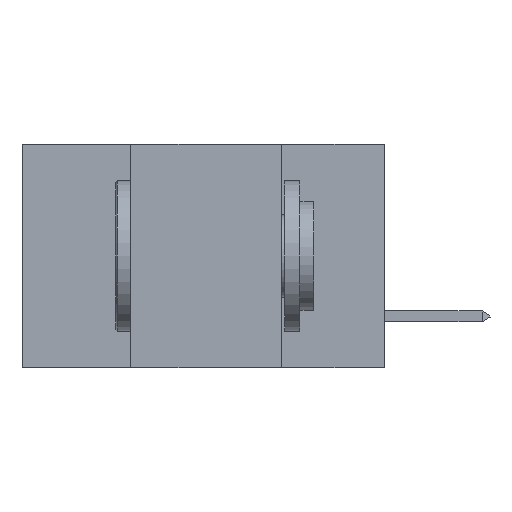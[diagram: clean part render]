
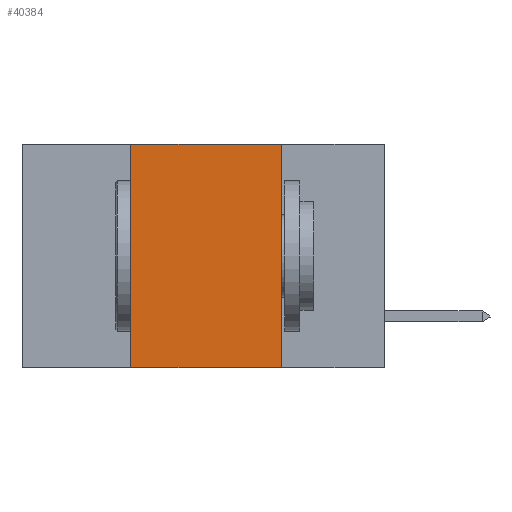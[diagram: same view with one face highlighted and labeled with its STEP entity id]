
A CAD part, left-side view. The second image highlights one B-rep face of the part: STEP entity #40384.
In plain terms, the highlighted planar face has unit normal (-1, 0, 0).
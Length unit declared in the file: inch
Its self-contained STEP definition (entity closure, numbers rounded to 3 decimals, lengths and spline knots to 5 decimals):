
#742 = ORIENTED_EDGE ( 'NONE', *, *, #41361, .F. ) ;
#785 = EDGE_LOOP ( 'NONE', ( #19359, #10120, #742, #43513 ) ) ;
#1730 = CARTESIAN_POINT ( 'NONE',  ( 0., 0.42, -0.37 ) ) ;
#3085 = LINE ( 'NONE', #10247, #39318 ) ;
#8878 = CARTESIAN_POINT ( 'NONE',  ( 0., 0.17, 0. ) ) ;
#9222 = DIRECTION ( 'NONE',  ( 0., -1., 0. ) ) ;
#9791 = VECTOR ( 'NONE', #37718, 39.37008 ) ;
#10120 = ORIENTED_EDGE ( 'NONE', *, *, #30629, .F. ) ;
#10247 = CARTESIAN_POINT ( 'NONE',  ( 0., 0.42, 0. ) ) ;
#11367 = VERTEX_POINT ( 'NONE', #8878 ) ;
#13706 = CARTESIAN_POINT ( 'NONE',  ( 0., 0.17, 0. ) ) ;
#13823 = VECTOR ( 'NONE', #42968, 39.37008 ) ;
#15061 = VERTEX_POINT ( 'NONE', #26260 ) ;
#15453 = CARTESIAN_POINT ( 'NONE',  ( 0., 0.6, -0.37 ) ) ;
#16656 = AXIS2_PLACEMENT_3D ( 'NONE', #32857, #35801, #36112 ) ;
#19359 = ORIENTED_EDGE ( 'NONE', *, *, #36199, .F. ) ;
#20117 = FACE_OUTER_BOUND ( 'NONE', #785, .T. ) ;
#24260 = LINE ( 'NONE', #15453, #13823 ) ;
#25712 = LINE ( 'NONE', #37942, #32861 ) ;
#26260 = CARTESIAN_POINT ( 'NONE',  ( 0., 0.17, -0.37 ) ) ;
#26929 = VERTEX_POINT ( 'NONE', #1730 ) ;
#28704 = PLANE ( 'NONE',  #16656 ) ;
#28743 = VERTEX_POINT ( 'NONE', #39030 ) ;
#30629 = EDGE_CURVE ( 'NONE', #28743, #11367, #25712, .T. ) ;
#32857 = CARTESIAN_POINT ( 'NONE',  ( 0., 0.6, 0. ) ) ;
#32861 = VECTOR ( 'NONE', #9222, 39.37008 ) ;
#35801 = DIRECTION ( 'NONE',  ( 1., 0., 0. ) ) ;
#36112 = DIRECTION ( 'NONE',  ( 0., 0., -1. ) ) ;
#36199 = EDGE_CURVE ( 'NONE', #11367, #15061, #43303, .T. ) ;
#37718 = DIRECTION ( 'NONE',  ( 0., 0., -1. ) ) ;
#37942 = CARTESIAN_POINT ( 'NONE',  ( 0., 0.6, 0. ) ) ;
#39030 = CARTESIAN_POINT ( 'NONE',  ( 0., 0.42, 0. ) ) ;
#39318 = VECTOR ( 'NONE', #45406, 39.37008 ) ;
#40384 = ADVANCED_FACE ( 'NONE', ( #20117 ), #28704, .F. ) ;
#41361 = EDGE_CURVE ( 'NONE', #26929, #28743, #3085, .T. ) ;
#42968 = DIRECTION ( 'NONE',  ( 0., -1., 0. ) ) ;
#43045 = EDGE_CURVE ( 'NONE', #26929, #15061, #24260, .T. ) ;
#43303 = LINE ( 'NONE', #13706, #9791 ) ;
#43513 = ORIENTED_EDGE ( 'NONE', *, *, #43045, .T. ) ;
#45406 = DIRECTION ( 'NONE',  ( 0., 0., 1. ) ) ;
